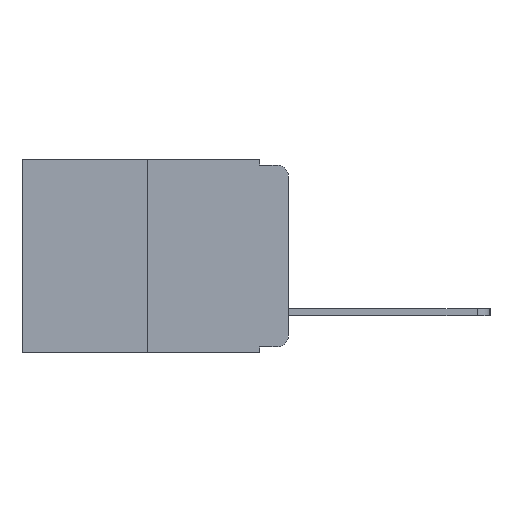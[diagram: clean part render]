
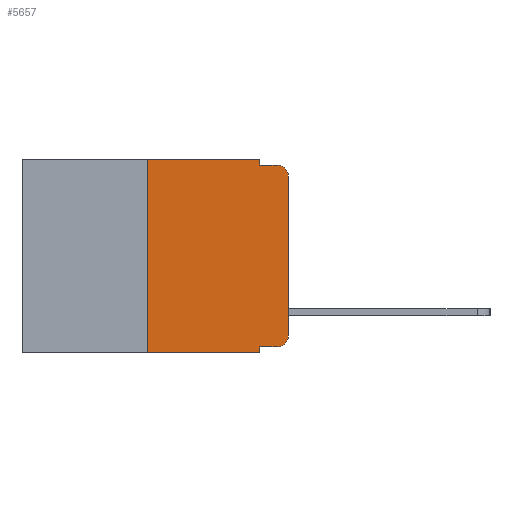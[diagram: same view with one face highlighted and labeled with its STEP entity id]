
A CAD part, left-side view. The second image highlights one B-rep face of the part: STEP entity #5657.
In plain terms, the highlighted planar face has unit normal (-1, 0, 0).
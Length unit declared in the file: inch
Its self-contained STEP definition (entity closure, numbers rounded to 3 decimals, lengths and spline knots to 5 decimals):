
#18 = ORIENTED_EDGE ( 'NONE', *, *, #13727, .F. ) ;
#82 = CARTESIAN_POINT ( 'NONE',  ( 0., 0.02, -0.03 ) ) ;
#142 = FACE_OUTER_BOUND ( 'NONE', #11360, .T. ) ;
#295 = VERTEX_POINT ( 'NONE', #23191 ) ;
#359 = VECTOR ( 'NONE', #15026, 39.37008 ) ;
#476 = VERTEX_POINT ( 'NONE', #16357 ) ;
#729 = LINE ( 'NONE', #5033, #14764 ) ;
#902 = DIRECTION ( 'NONE',  ( 0., 0., 1. ) ) ;
#1356 = CIRCLE ( 'NONE', #13820, 0.02 ) ;
#1540 = VERTEX_POINT ( 'NONE', #12363 ) ;
#1574 = VERTEX_POINT ( 'NONE', #23564 ) ;
#1978 = DIRECTION ( 'NONE',  ( 0., 0., -1. ) ) ;
#2070 = DIRECTION ( 'NONE',  ( 0., 0., 1. ) ) ;
#2206 = PLANE ( 'NONE',  #21473 ) ;
#2281 = VERTEX_POINT ( 'NONE', #9325 ) ;
#2744 = DIRECTION ( 'NONE',  ( 0., -1., 0. ) ) ;
#2756 = CARTESIAN_POINT ( 'NONE',  ( 0., 0.25, 0. ) ) ;
#3801 = EDGE_CURVE ( 'NONE', #19705, #476, #22580, .T. ) ;
#4557 = CARTESIAN_POINT ( 'NONE',  ( 0., 0.473, 0. ) ) ;
#5033 = CARTESIAN_POINT ( 'NONE',  ( 0., 0.051, 0. ) ) ;
#5135 = EDGE_CURVE ( 'NONE', #295, #7101, #1356, .T. ) ;
#5244 = LINE ( 'NONE', #11214, #359 ) ;
#5616 = CARTESIAN_POINT ( 'NONE',  ( 0., 0.051, 0. ) ) ;
#5657 = ADVANCED_FACE ( 'NONE', ( #142 ), #2206, .F. ) ;
#5658 = VECTOR ( 'NONE', #902, 39.37008 ) ;
#5722 = CARTESIAN_POINT ( 'NONE',  ( 0., 0.25, 0. ) ) ;
#5838 = DIRECTION ( 'NONE',  ( -1., 0., 0. ) ) ;
#6268 = ORIENTED_EDGE ( 'NONE', *, *, #18627, .T. ) ;
#6347 = ORIENTED_EDGE ( 'NONE', *, *, #8812, .F. ) ;
#6518 = ORIENTED_EDGE ( 'NONE', *, *, #3801, .T. ) ;
#7101 = VERTEX_POINT ( 'NONE', #23605 ) ;
#7466 = ORIENTED_EDGE ( 'NONE', *, *, #5135, .T. ) ;
#7564 = EDGE_CURVE ( 'NONE', #1540, #295, #5244, .T. ) ;
#7898 = VERTEX_POINT ( 'NONE', #2756 ) ;
#8365 = VECTOR ( 'NONE', #9220, 39.37008 ) ;
#8385 = CIRCLE ( 'NONE', #10607, 0.02 ) ;
#8671 = VERTEX_POINT ( 'NONE', #17860 ) ;
#8812 = EDGE_CURVE ( 'NONE', #1540, #476, #13226, .T. ) ;
#9047 = ORIENTED_EDGE ( 'NONE', *, *, #7564, .T. ) ;
#9220 = DIRECTION ( 'NONE',  ( 0., 0., -1. ) ) ;
#9325 = CARTESIAN_POINT ( 'NONE',  ( 0., 0., -0.03 ) ) ;
#9655 = ORIENTED_EDGE ( 'NONE', *, *, #14960, .T. ) ;
#9760 = DIRECTION ( 'NONE',  ( 0., -1., 0. ) ) ;
#10087 = EDGE_CURVE ( 'NONE', #19705, #7898, #17141, .T. ) ;
#10607 = AXIS2_PLACEMENT_3D ( 'NONE', #82, #12946, #1978 ) ;
#10663 = VERTEX_POINT ( 'NONE', #5616 ) ;
#11214 = CARTESIAN_POINT ( 'NONE',  ( 0., 0.051, -0.333 ) ) ;
#11360 = EDGE_LOOP ( 'NONE', ( #6268, #9655, #18, #23377, #12503, #12811, #6518, #6347, #9047, #7466 ) ) ;
#11587 = LINE ( 'NONE', #13106, #15857 ) ;
#12284 = VECTOR ( 'NONE', #2070, 39.37008 ) ;
#12363 = CARTESIAN_POINT ( 'NONE',  ( 0., 0.051, -0.333 ) ) ;
#12497 = EDGE_CURVE ( 'NONE', #10663, #1574, #729, .T. ) ;
#12503 = ORIENTED_EDGE ( 'NONE', *, *, #18007, .F. ) ;
#12811 = ORIENTED_EDGE ( 'NONE', *, *, #10087, .F. ) ;
#12946 = DIRECTION ( 'NONE',  ( -1., 0., 0. ) ) ;
#13106 = CARTESIAN_POINT ( 'NONE',  ( 0., 0.051, -0.01 ) ) ;
#13226 = LINE ( 'NONE', #20147, #8365 ) ;
#13425 = VECTOR ( 'NONE', #2744, 39.37008 ) ;
#13727 = EDGE_CURVE ( 'NONE', #1574, #8671, #11587, .T. ) ;
#13820 = AXIS2_PLACEMENT_3D ( 'NONE', #16784, #5838, #20464 ) ;
#14764 = VECTOR ( 'NONE', #15990, 39.37008 ) ;
#14960 = EDGE_CURVE ( 'NONE', #2281, #8671, #8385, .T. ) ;
#14994 = CARTESIAN_POINT ( 'NONE',  ( 0., 0.473, 0. ) ) ;
#15026 = DIRECTION ( 'NONE',  ( 0., -1., 0. ) ) ;
#15857 = VECTOR ( 'NONE', #16768, 39.37008 ) ;
#15990 = DIRECTION ( 'NONE',  ( 0., 0., -1. ) ) ;
#16357 = CARTESIAN_POINT ( 'NONE',  ( 0., 0.051, -0.343 ) ) ;
#16768 = DIRECTION ( 'NONE',  ( 0., -1., 0. ) ) ;
#16784 = CARTESIAN_POINT ( 'NONE',  ( 0., 0.02, -0.313 ) ) ;
#17141 = LINE ( 'NONE', #5722, #12284 ) ;
#17747 = VECTOR ( 'NONE', #9760, 39.37008 ) ;
#17860 = CARTESIAN_POINT ( 'NONE',  ( 0., 0.02, -0.01 ) ) ;
#18007 = EDGE_CURVE ( 'NONE', #7898, #10663, #23085, .T. ) ;
#18254 = CARTESIAN_POINT ( 'NONE',  ( 0., 0.473, -0.343 ) ) ;
#18627 = EDGE_CURVE ( 'NONE', #7101, #2281, #20234, .T. ) ;
#19705 = VERTEX_POINT ( 'NONE', #20538 ) ;
#20147 = CARTESIAN_POINT ( 'NONE',  ( 0., 0.051, 0. ) ) ;
#20234 = LINE ( 'NONE', #22773, #5658 ) ;
#20464 = DIRECTION ( 'NONE',  ( 0., 0., -1. ) ) ;
#20538 = CARTESIAN_POINT ( 'NONE',  ( 0., 0.25, -0.343 ) ) ;
#21473 = AXIS2_PLACEMENT_3D ( 'NONE', #14994, #23506, #22438 ) ;
#22438 = DIRECTION ( 'NONE',  ( 0., 0., -1. ) ) ;
#22580 = LINE ( 'NONE', #18254, #17747 ) ;
#22773 = CARTESIAN_POINT ( 'NONE',  ( 0., 0., 0. ) ) ;
#23085 = LINE ( 'NONE', #4557, #13425 ) ;
#23191 = CARTESIAN_POINT ( 'NONE',  ( 0., 0.02, -0.333 ) ) ;
#23377 = ORIENTED_EDGE ( 'NONE', *, *, #12497, .F. ) ;
#23506 = DIRECTION ( 'NONE',  ( 1., 0., 0. ) ) ;
#23564 = CARTESIAN_POINT ( 'NONE',  ( 0., 0.051, -0.01 ) ) ;
#23605 = CARTESIAN_POINT ( 'NONE',  ( 0., 0., -0.313 ) ) ;
